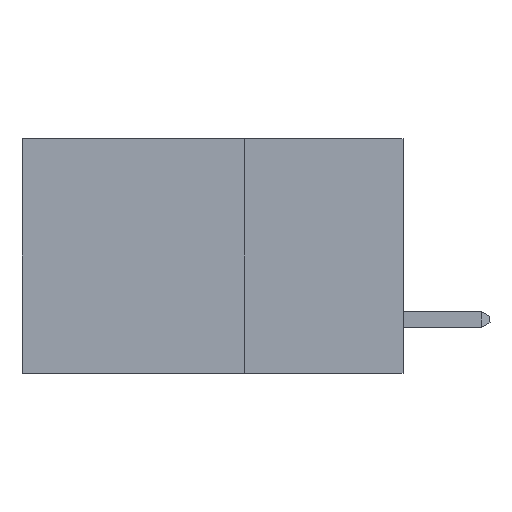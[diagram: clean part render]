
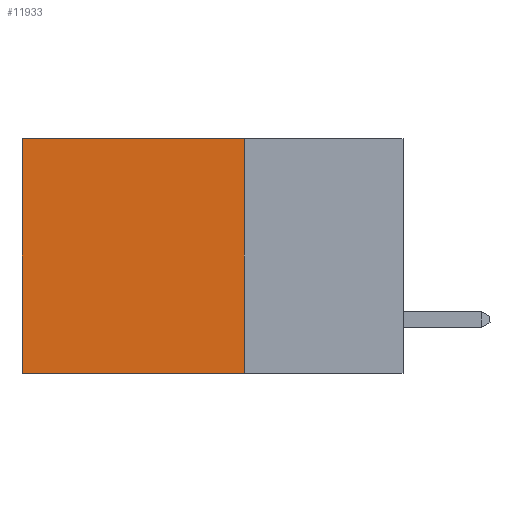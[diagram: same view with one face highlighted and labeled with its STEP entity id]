
A CAD part, left-side view. The second image highlights one B-rep face of the part: STEP entity #11933.
In plain terms, the highlighted planar face has unit normal (-1, 0, 0).
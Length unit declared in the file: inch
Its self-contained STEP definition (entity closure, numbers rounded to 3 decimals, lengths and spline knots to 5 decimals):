
#831 = VERTEX_POINT ( 'NONE', #2397 ) ;
#902 = CARTESIAN_POINT ( 'NONE',  ( 0.2875, 0.6, -0.37 ) ) ;
#1366 = EDGE_CURVE ( 'NONE', #2699, #19440, #8337, .T. ) ;
#2397 = CARTESIAN_POINT ( 'NONE',  ( 0.2875, 0.25, -0.37 ) ) ;
#2699 = VERTEX_POINT ( 'NONE', #18684 ) ;
#3059 = EDGE_CURVE ( 'NONE', #831, #4393, #22780, .T. ) ;
#3331 = CARTESIAN_POINT ( 'NONE',  ( 0.2875, 0.25, 0. ) ) ;
#3547 = AXIS2_PLACEMENT_3D ( 'NONE', #9101, #22361, #11056 ) ;
#4393 = VERTEX_POINT ( 'NONE', #902 ) ;
#6157 = CARTESIAN_POINT ( 'NONE',  ( 0.2875, 0.25, -0.37 ) ) ;
#7820 = CARTESIAN_POINT ( 'NONE',  ( 0.2875, 0.25, 0. ) ) ;
#8337 = LINE ( 'NONE', #7820, #22297 ) ;
#9101 = CARTESIAN_POINT ( 'NONE',  ( 0.2875, 0.25, 0. ) ) ;
#9108 = DIRECTION ( 'NONE',  ( 0., 0., -1. ) ) ;
#10137 = DIRECTION ( 'NONE',  ( 0., 1., 0. ) ) ;
#10283 = ORIENTED_EDGE ( 'NONE', *, *, #20713, .T. ) ;
#10979 = PLANE ( 'NONE',  #3547 ) ;
#11056 = DIRECTION ( 'NONE',  ( 0., 0., -1. ) ) ;
#11625 = LINE ( 'NONE', #3331, #17309 ) ;
#11895 = CARTESIAN_POINT ( 'NONE',  ( 0.2875, 0.6, 0. ) ) ;
#11933 = ADVANCED_FACE ( 'NONE', ( #23507 ), #10979, .F. ) ;
#13825 = DIRECTION ( 'NONE',  ( 0., 0., -1. ) ) ;
#13843 = EDGE_CURVE ( 'NONE', #2699, #831, #11625, .T. ) ;
#15219 = LINE ( 'NONE', #11895, #24580 ) ;
#16366 = CARTESIAN_POINT ( 'NONE',  ( 0.2875, 0.6, 0. ) ) ;
#17309 = VECTOR ( 'NONE', #9108, 39.37008 ) ;
#17856 = VECTOR ( 'NONE', #10137, 39.37008 ) ;
#17900 = ORIENTED_EDGE ( 'NONE', *, *, #13843, .F. ) ;
#18522 = DIRECTION ( 'NONE',  ( 0., 1., 0. ) ) ;
#18684 = CARTESIAN_POINT ( 'NONE',  ( 0.2875, 0.25, 0. ) ) ;
#18905 = ORIENTED_EDGE ( 'NONE', *, *, #3059, .F. ) ;
#19440 = VERTEX_POINT ( 'NONE', #16366 ) ;
#20713 = EDGE_CURVE ( 'NONE', #19440, #4393, #15219, .T. ) ;
#20804 = ORIENTED_EDGE ( 'NONE', *, *, #1366, .T. ) ;
#22297 = VECTOR ( 'NONE', #18522, 39.37008 ) ;
#22354 = EDGE_LOOP ( 'NONE', ( #10283, #18905, #17900, #20804 ) ) ;
#22361 = DIRECTION ( 'NONE',  ( 1., 0., 0. ) ) ;
#22780 = LINE ( 'NONE', #6157, #17856 ) ;
#23507 = FACE_OUTER_BOUND ( 'NONE', #22354, .T. ) ;
#24580 = VECTOR ( 'NONE', #13825, 39.37008 ) ;
